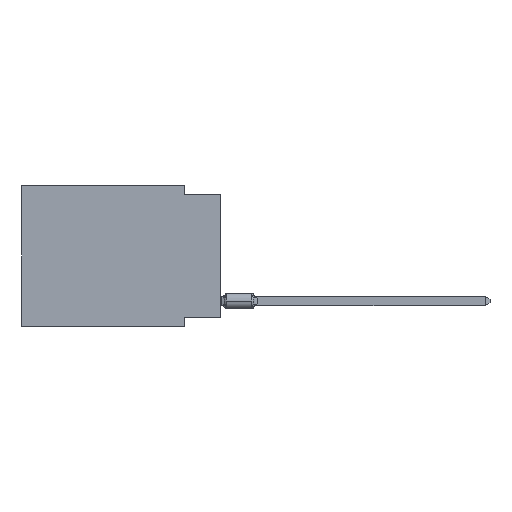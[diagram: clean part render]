
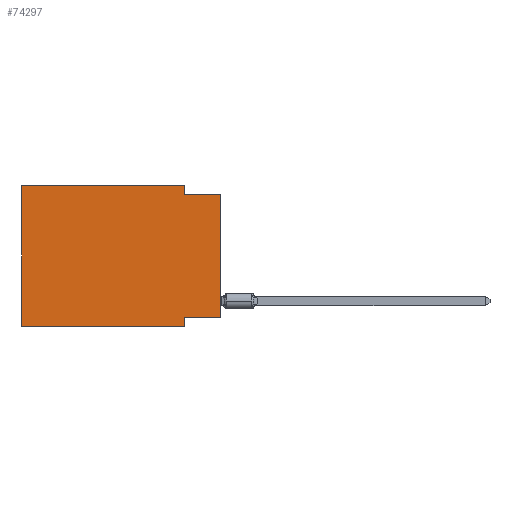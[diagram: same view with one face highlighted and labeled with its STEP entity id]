
A CAD part, left-side view. The second image highlights one B-rep face of the part: STEP entity #74297.
In plain terms, the highlighted planar face has unit normal (-1, 0, 0).
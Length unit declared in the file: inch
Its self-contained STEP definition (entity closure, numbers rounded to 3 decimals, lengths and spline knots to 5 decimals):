
#1136 = CARTESIAN_POINT ( 'NONE',  ( 0., 0.55, 0. ) ) ;
#1543 = LINE ( 'NONE', #1136, #42806 ) ;
#1984 = DIRECTION ( 'NONE',  ( 0., -1., 0. ) ) ;
#3376 = CARTESIAN_POINT ( 'NONE',  ( 0., 0., -0.365 ) ) ;
#6498 = CARTESIAN_POINT ( 'NONE',  ( 0., 0.55, -0.39 ) ) ;
#8084 = ORIENTED_EDGE ( 'NONE', *, *, #31610, .F. ) ;
#8776 = DIRECTION ( 'NONE',  ( 0., 0., 1. ) ) ;
#9585 = VERTEX_POINT ( 'NONE', #64476 ) ;
#13524 = VERTEX_POINT ( 'NONE', #36946 ) ;
#14843 = CARTESIAN_POINT ( 'NONE',  ( 0., 0., 0. ) ) ;
#15885 = LINE ( 'NONE', #3376, #29488 ) ;
#16057 = DIRECTION ( 'NONE',  ( 0., 0., 1. ) ) ;
#16837 = VECTOR ( 'NONE', #1984, 39.37008 ) ;
#17337 = VECTOR ( 'NONE', #19419, 39.37008 ) ;
#19419 = DIRECTION ( 'NONE',  ( 0., -1., 0. ) ) ;
#19501 = ORIENTED_EDGE ( 'NONE', *, *, #49584, .F. ) ;
#22652 = VECTOR ( 'NONE', #16057, 39.37008 ) ;
#24814 = ORIENTED_EDGE ( 'NONE', *, *, #41549, .F. ) ;
#25343 = CARTESIAN_POINT ( 'NONE',  ( 0., 0.1, -0.39 ) ) ;
#26694 = LINE ( 'NONE', #52135, #51020 ) ;
#26816 = CARTESIAN_POINT ( 'NONE',  ( 0., 0., -0.025 ) ) ;
#27140 = ORIENTED_EDGE ( 'NONE', *, *, #61255, .T. ) ;
#27282 = CARTESIAN_POINT ( 'NONE',  ( 0., 0.55, 0. ) ) ;
#29488 = VECTOR ( 'NONE', #34062, 39.37008 ) ;
#30440 = EDGE_CURVE ( 'NONE', #9585, #13524, #15885, .T. ) ;
#30894 = ORIENTED_EDGE ( 'NONE', *, *, #30440, .F. ) ;
#31610 = EDGE_CURVE ( 'NONE', #65477, #33756, #50866, .T. ) ;
#32290 = VECTOR ( 'NONE', #79243, 39.37008 ) ;
#33756 = VERTEX_POINT ( 'NONE', #26816 ) ;
#34062 = DIRECTION ( 'NONE',  ( 0., 1., 0. ) ) ;
#34372 = VERTEX_POINT ( 'NONE', #25343 ) ;
#35721 = VERTEX_POINT ( 'NONE', #53624 ) ;
#36946 = CARTESIAN_POINT ( 'NONE',  ( 0., 0.1, -0.365 ) ) ;
#37929 = EDGE_LOOP ( 'NONE', ( #27140, #8084, #19501, #44610, #67318, #71237, #24814, #30894 ) ) ;
#38357 = EDGE_CURVE ( 'NONE', #46903, #34372, #38762, .T. ) ;
#38762 = LINE ( 'NONE', #6498, #17337 ) ;
#40534 = DIRECTION ( 'NONE',  ( 0., 0., -1. ) ) ;
#41479 = LINE ( 'NONE', #66135, #22652 ) ;
#41549 = EDGE_CURVE ( 'NONE', #13524, #34372, #26694, .T. ) ;
#42806 = VECTOR ( 'NONE', #52011, 39.37008 ) ;
#44610 = ORIENTED_EDGE ( 'NONE', *, *, #71360, .F. ) ;
#45541 = LINE ( 'NONE', #14843, #79142 ) ;
#46903 = VERTEX_POINT ( 'NONE', #63823 ) ;
#49584 = EDGE_CURVE ( 'NONE', #35721, #65477, #60664, .T. ) ;
#50866 = LINE ( 'NONE', #75516, #16837 ) ;
#51020 = VECTOR ( 'NONE', #51350, 39.37008 ) ;
#51350 = DIRECTION ( 'NONE',  ( 0., 0., -1. ) ) ;
#52011 = DIRECTION ( 'NONE',  ( 0., -1., 0. ) ) ;
#52135 = CARTESIAN_POINT ( 'NONE',  ( 0., 0.1, -0.39 ) ) ;
#53624 = CARTESIAN_POINT ( 'NONE',  ( 0., 0.1, 0. ) ) ;
#57177 = CARTESIAN_POINT ( 'NONE',  ( 0., 0.55, 0. ) ) ;
#57706 = EDGE_CURVE ( 'NONE', #46903, #69438, #41479, .T. ) ;
#58753 = PLANE ( 'NONE',  #73253 ) ;
#59465 = CARTESIAN_POINT ( 'NONE',  ( 0., 0.1, 0. ) ) ;
#60664 = LINE ( 'NONE', #59465, #32290 ) ;
#61255 = EDGE_CURVE ( 'NONE', #9585, #33756, #45541, .T. ) ;
#63823 = CARTESIAN_POINT ( 'NONE',  ( 0., 0.55, -0.39 ) ) ;
#64476 = CARTESIAN_POINT ( 'NONE',  ( 0., 0., -0.365 ) ) ;
#64721 = CARTESIAN_POINT ( 'NONE',  ( 0., 0.1, -0.025 ) ) ;
#65191 = DIRECTION ( 'NONE',  ( 1., 0., 0. ) ) ;
#65477 = VERTEX_POINT ( 'NONE', #64721 ) ;
#66135 = CARTESIAN_POINT ( 'NONE',  ( 0., 0.55, 0. ) ) ;
#67318 = ORIENTED_EDGE ( 'NONE', *, *, #57706, .F. ) ;
#69438 = VERTEX_POINT ( 'NONE', #27282 ) ;
#71237 = ORIENTED_EDGE ( 'NONE', *, *, #38357, .T. ) ;
#71360 = EDGE_CURVE ( 'NONE', #69438, #35721, #1543, .T. ) ;
#73253 = AXIS2_PLACEMENT_3D ( 'NONE', #57177, #65191, #40534 ) ;
#74297 = ADVANCED_FACE ( 'NONE', ( #76932 ), #58753, .F. ) ;
#75516 = CARTESIAN_POINT ( 'NONE',  ( 0., 0., -0.025 ) ) ;
#76932 = FACE_OUTER_BOUND ( 'NONE', #37929, .T. ) ;
#79142 = VECTOR ( 'NONE', #8776, 39.37008 ) ;
#79243 = DIRECTION ( 'NONE',  ( 0., 0., -1. ) ) ;
